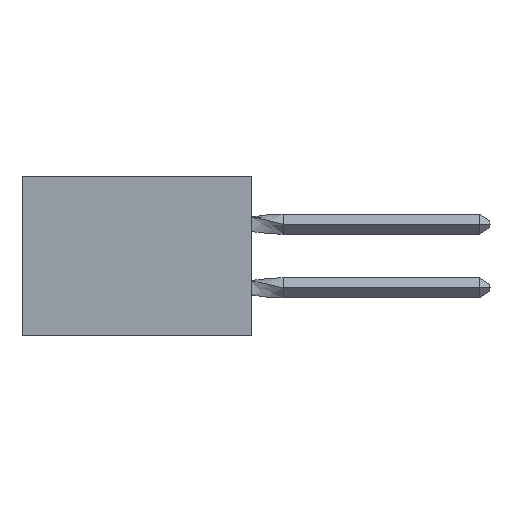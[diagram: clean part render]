
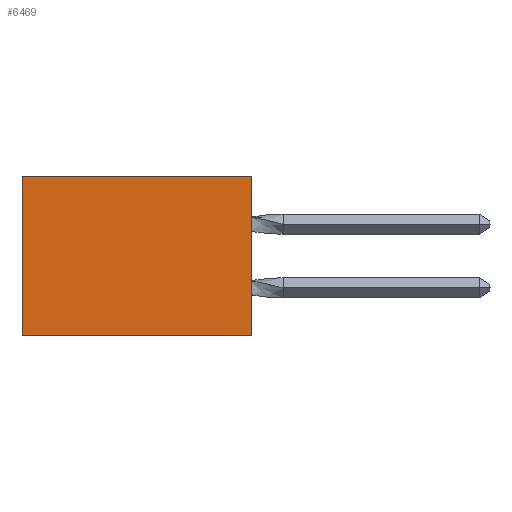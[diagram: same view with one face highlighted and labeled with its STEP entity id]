
A CAD part, left-side view. The second image highlights one B-rep face of the part: STEP entity #6469.
In plain terms, the highlighted planar face has unit normal (-1, 0, 0).
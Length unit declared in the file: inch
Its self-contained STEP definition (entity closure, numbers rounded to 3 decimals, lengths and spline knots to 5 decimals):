
#56 = CARTESIAN_POINT ( 'NONE',  ( 0.305, 0.72, -0.5 ) ) ;
#205 = CARTESIAN_POINT ( 'NONE',  ( 0.305, 0.72, -0.5 ) ) ;
#921 = EDGE_LOOP ( 'NONE', ( #15818, #14248, #7759, #9562 ) ) ;
#1628 = DIRECTION ( 'NONE',  ( 0., 0., -1. ) ) ;
#2016 = CARTESIAN_POINT ( 'NONE',  ( 0.305, 0., 0. ) ) ;
#2083 = EDGE_CURVE ( 'NONE', #5664, #13225, #2450, .T. ) ;
#2149 = EDGE_CURVE ( 'NONE', #5664, #17256, #18333, .T. ) ;
#2450 = LINE ( 'NONE', #7061, #4223 ) ;
#3131 = VECTOR ( 'NONE', #12859, 39.37008 ) ;
#3189 = EDGE_CURVE ( 'NONE', #17256, #5816, #8713, .T. ) ;
#4223 = VECTOR ( 'NONE', #4327, 39.37008 ) ;
#4327 = DIRECTION ( 'NONE',  ( 0., 0., -1. ) ) ;
#4519 = CARTESIAN_POINT ( 'NONE',  ( 0.305, 0., -0.5 ) ) ;
#4802 = CARTESIAN_POINT ( 'NONE',  ( 0.305, 0., -0.5 ) ) ;
#5664 = VERTEX_POINT ( 'NONE', #8118 ) ;
#5816 = VERTEX_POINT ( 'NONE', #205 ) ;
#6469 = ADVANCED_FACE ( 'NONE', ( #10231 ), #7329, .F. ) ;
#7013 = CARTESIAN_POINT ( 'NONE',  ( 0.305, 0.72, 0. ) ) ;
#7061 = CARTESIAN_POINT ( 'NONE',  ( 0.305, 0., -0.5 ) ) ;
#7329 = PLANE ( 'NONE',  #13635 ) ;
#7759 = ORIENTED_EDGE ( 'NONE', *, *, #2083, .F. ) ;
#8118 = CARTESIAN_POINT ( 'NONE',  ( 0.305, 0., 0. ) ) ;
#8500 = VECTOR ( 'NONE', #12996, 39.37008 ) ;
#8713 = LINE ( 'NONE', #56, #8500 ) ;
#9562 = ORIENTED_EDGE ( 'NONE', *, *, #2149, .T. ) ;
#10107 = EDGE_CURVE ( 'NONE', #13225, #5816, #15181, .T. ) ;
#10231 = FACE_OUTER_BOUND ( 'NONE', #921, .T. ) ;
#12859 = DIRECTION ( 'NONE',  ( 0., 1., 0. ) ) ;
#12996 = DIRECTION ( 'NONE',  ( 0., 0., -1. ) ) ;
#13225 = VERTEX_POINT ( 'NONE', #4802 ) ;
#13635 = AXIS2_PLACEMENT_3D ( 'NONE', #4519, #17619, #1628 ) ;
#14248 = ORIENTED_EDGE ( 'NONE', *, *, #10107, .F. ) ;
#14429 = CARTESIAN_POINT ( 'NONE',  ( 0.305, 0., -0.5 ) ) ;
#14478 = VECTOR ( 'NONE', #17800, 39.37008 ) ;
#15181 = LINE ( 'NONE', #14429, #3131 ) ;
#15818 = ORIENTED_EDGE ( 'NONE', *, *, #3189, .T. ) ;
#17256 = VERTEX_POINT ( 'NONE', #7013 ) ;
#17619 = DIRECTION ( 'NONE',  ( 1., 0., 0. ) ) ;
#17800 = DIRECTION ( 'NONE',  ( 0., 1., 0. ) ) ;
#18333 = LINE ( 'NONE', #2016, #14478 ) ;
